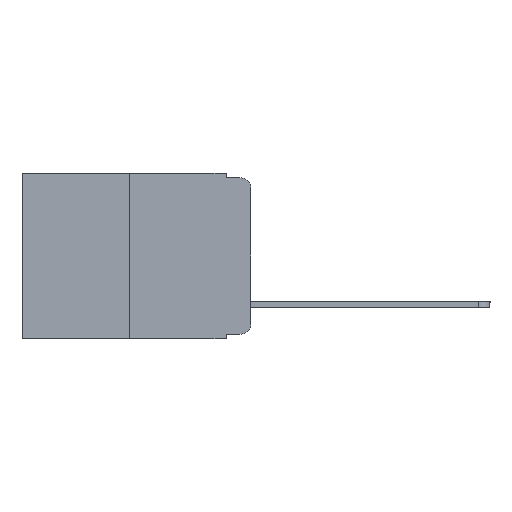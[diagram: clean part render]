
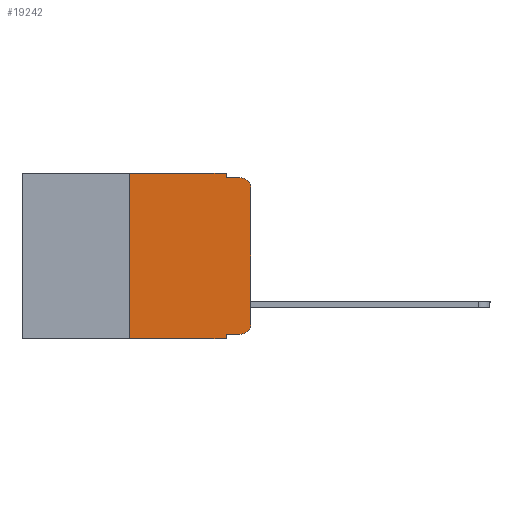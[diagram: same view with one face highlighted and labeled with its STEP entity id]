
A CAD part, left-side view. The second image highlights one B-rep face of the part: STEP entity #19242.
In plain terms, the highlighted planar face has unit normal (-1, 0, 0).
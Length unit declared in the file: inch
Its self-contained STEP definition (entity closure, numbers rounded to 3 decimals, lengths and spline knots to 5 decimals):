
#146 = VECTOR ( 'NONE', #3851, 39.37008 ) ;
#153 = CARTESIAN_POINT ( 'NONE',  ( 0., 0.051, -0.333 ) ) ;
#194 = EDGE_CURVE ( 'NONE', #10350, #13307, #1757, .T. ) ;
#481 = CARTESIAN_POINT ( 'NONE',  ( 0., 0.473, -0.343 ) ) ;
#541 = ORIENTED_EDGE ( 'NONE', *, *, #8902, .F. ) ;
#745 = CARTESIAN_POINT ( 'NONE',  ( 0., 0.02, -0.333 ) ) ;
#915 = DIRECTION ( 'NONE',  ( 0., -1., 0. ) ) ;
#1336 = CARTESIAN_POINT ( 'NONE',  ( 0., 0.25, -0.343 ) ) ;
#1757 = LINE ( 'NONE', #481, #12566 ) ;
#2327 = DIRECTION ( 'NONE',  ( 0., 0., 1. ) ) ;
#2867 = EDGE_CURVE ( 'NONE', #9383, #15722, #8621, .T. ) ;
#2984 = EDGE_CURVE ( 'NONE', #13889, #12290, #18551, .T. ) ;
#3702 = DIRECTION ( 'NONE',  ( -1., 0., 0. ) ) ;
#3851 = DIRECTION ( 'NONE',  ( 0., -1., 0. ) ) ;
#3986 = DIRECTION ( 'NONE',  ( 0., 0., -1. ) ) ;
#4394 = VERTEX_POINT ( 'NONE', #6821 ) ;
#4962 = DIRECTION ( 'NONE',  ( -1., 0., 0. ) ) ;
#5312 = CARTESIAN_POINT ( 'NONE',  ( 0., 0., -0.03 ) ) ;
#5533 = CARTESIAN_POINT ( 'NONE',  ( 0., 0.02, -0.03 ) ) ;
#5747 = EDGE_CURVE ( 'NONE', #10350, #8742, #20168, .T. ) ;
#6207 = CARTESIAN_POINT ( 'NONE',  ( 0., 0.473, 0. ) ) ;
#6224 = PLANE ( 'NONE',  #16742 ) ;
#6297 = ORIENTED_EDGE ( 'NONE', *, *, #19975, .T. ) ;
#6756 = ORIENTED_EDGE ( 'NONE', *, *, #194, .T. ) ;
#6821 = CARTESIAN_POINT ( 'NONE',  ( 0., 0.051, -0.333 ) ) ;
#7041 = CARTESIAN_POINT ( 'NONE',  ( 0., 0.02, -0.01 ) ) ;
#7187 = LINE ( 'NONE', #153, #146 ) ;
#7224 = ORIENTED_EDGE ( 'NONE', *, *, #2984, .T. ) ;
#7700 = ORIENTED_EDGE ( 'NONE', *, *, #8770, .F. ) ;
#7810 = CARTESIAN_POINT ( 'NONE',  ( 0., 0.051, 0. ) ) ;
#7843 = VECTOR ( 'NONE', #14252, 39.37008 ) ;
#8545 = DIRECTION ( 'NONE',  ( 0., 0., -1. ) ) ;
#8621 = CIRCLE ( 'NONE', #21856, 0.02 ) ;
#8726 = CARTESIAN_POINT ( 'NONE',  ( 0., 0.051, -0.01 ) ) ;
#8742 = VERTEX_POINT ( 'NONE', #16440 ) ;
#8770 = EDGE_CURVE ( 'NONE', #13136, #12290, #10782, .T. ) ;
#8902 = EDGE_CURVE ( 'NONE', #12863, #13136, #16559, .T. ) ;
#9383 = VERTEX_POINT ( 'NONE', #745 ) ;
#9682 = CARTESIAN_POINT ( 'NONE',  ( 0., 0.25, 0. ) ) ;
#9965 = VECTOR ( 'NONE', #915, 39.37008 ) ;
#10140 = ORIENTED_EDGE ( 'NONE', *, *, #18060, .F. ) ;
#10153 = CARTESIAN_POINT ( 'NONE',  ( 0., 0.02, -0.313 ) ) ;
#10350 = VERTEX_POINT ( 'NONE', #1336 ) ;
#10398 = EDGE_CURVE ( 'NONE', #4394, #9383, #7187, .T. ) ;
#10782 = LINE ( 'NONE', #12519, #7843 ) ;
#11441 = EDGE_CURVE ( 'NONE', #8742, #12863, #18322, .T. ) ;
#11596 = VECTOR ( 'NONE', #3986, 39.37008 ) ;
#11649 = EDGE_LOOP ( 'NONE', ( #6297, #7224, #7700, #541, #16506, #13549, #6756, #10140, #17412, #16450 ) ) ;
#12278 = CARTESIAN_POINT ( 'NONE',  ( 0., 0.051, 0. ) ) ;
#12290 = VERTEX_POINT ( 'NONE', #7041 ) ;
#12519 = CARTESIAN_POINT ( 'NONE',  ( 0., 0.051, -0.01 ) ) ;
#12566 = VECTOR ( 'NONE', #22340, 39.37008 ) ;
#12693 = LINE ( 'NONE', #18124, #14186 ) ;
#12863 = VERTEX_POINT ( 'NONE', #15515 ) ;
#13136 = VERTEX_POINT ( 'NONE', #8726 ) ;
#13249 = DIRECTION ( 'NONE',  ( 0., 0., -1. ) ) ;
#13307 = VERTEX_POINT ( 'NONE', #16879 ) ;
#13549 = ORIENTED_EDGE ( 'NONE', *, *, #5747, .F. ) ;
#13889 = VERTEX_POINT ( 'NONE', #5312 ) ;
#14186 = VECTOR ( 'NONE', #2327, 39.37008 ) ;
#14252 = DIRECTION ( 'NONE',  ( 0., -1., 0. ) ) ;
#14813 = DIRECTION ( 'NONE',  ( 0., 0., -1. ) ) ;
#15311 = FACE_OUTER_BOUND ( 'NONE', #11649, .T. ) ;
#15515 = CARTESIAN_POINT ( 'NONE',  ( 0., 0.051, 0. ) ) ;
#15722 = VERTEX_POINT ( 'NONE', #20655 ) ;
#15961 = LINE ( 'NONE', #12278, #11596 ) ;
#16440 = CARTESIAN_POINT ( 'NONE',  ( 0., 0.25, 0. ) ) ;
#16450 = ORIENTED_EDGE ( 'NONE', *, *, #2867, .T. ) ;
#16506 = ORIENTED_EDGE ( 'NONE', *, *, #11441, .F. ) ;
#16559 = LINE ( 'NONE', #7810, #18129 ) ;
#16742 = AXIS2_PLACEMENT_3D ( 'NONE', #22355, #18872, #13249 ) ;
#16879 = CARTESIAN_POINT ( 'NONE',  ( 0., 0.051, -0.343 ) ) ;
#17412 = ORIENTED_EDGE ( 'NONE', *, *, #10398, .T. ) ;
#18060 = EDGE_CURVE ( 'NONE', #4394, #13307, #15961, .T. ) ;
#18124 = CARTESIAN_POINT ( 'NONE',  ( 0., 0., 0. ) ) ;
#18129 = VECTOR ( 'NONE', #14813, 39.37008 ) ;
#18322 = LINE ( 'NONE', #6207, #9965 ) ;
#18551 = CIRCLE ( 'NONE', #21102, 0.02 ) ;
#18872 = DIRECTION ( 'NONE',  ( 1., 0., 0. ) ) ;
#19242 = ADVANCED_FACE ( 'NONE', ( #15311 ), #6224, .F. ) ;
#19975 = EDGE_CURVE ( 'NONE', #15722, #13889, #12693, .T. ) ;
#20168 = LINE ( 'NONE', #9682, #20427 ) ;
#20427 = VECTOR ( 'NONE', #21789, 39.37008 ) ;
#20655 = CARTESIAN_POINT ( 'NONE',  ( 0., 0., -0.313 ) ) ;
#21102 = AXIS2_PLACEMENT_3D ( 'NONE', #5533, #3702, #21430 ) ;
#21430 = DIRECTION ( 'NONE',  ( 0., 0., -1. ) ) ;
#21789 = DIRECTION ( 'NONE',  ( 0., 0., 1. ) ) ;
#21856 = AXIS2_PLACEMENT_3D ( 'NONE', #10153, #4962, #8545 ) ;
#22340 = DIRECTION ( 'NONE',  ( 0., -1., 0. ) ) ;
#22355 = CARTESIAN_POINT ( 'NONE',  ( 0., 0.473, 0. ) ) ;
